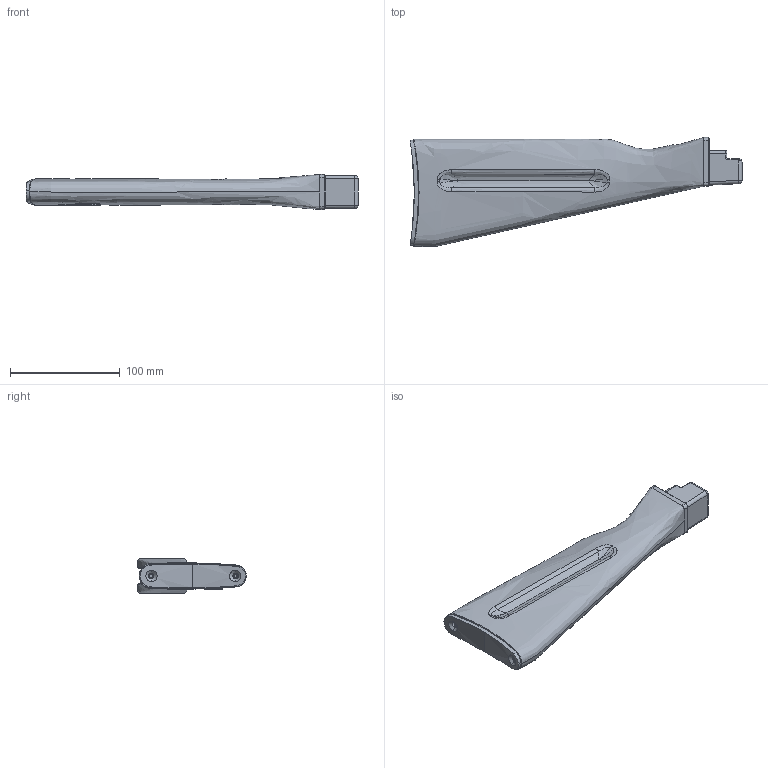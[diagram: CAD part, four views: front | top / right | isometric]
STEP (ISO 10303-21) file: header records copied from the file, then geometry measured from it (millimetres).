
FILE_DESCRIPTION (( 'STEP AP214' ), '1' );
FILE_NAME ('AK_Stock.STEP', '2013-10-08T06:17:21', ( 'elpi' ), ( '' ), 'SwSTEP 2.0', 'SolidWorks 2013', '' );
FILE_SCHEMA (( 'AUTOMOTIVE_DESIGN' ));
Length unit declared in the file: millimetre
Products named in the file (1): AK_Stock
Bounding box: 303 x 99.5 x 32 mm (x, y, z)
Volume: 405047.4 mm3; surface area: 53722.4 mm2
Topology: 1 solids, 1 shells, 163 faces, 379 edges, 228 vertices
Faces by surface type: bspline 53, cylinder 53, plane 36, torus 13, cone 6, sphere 2
Entity records: 12363 total; most frequent: CARTESIAN_POINT 8993, ORIENTED_EDGE 754, DIRECTION 603, EDGE_CURVE 377, AXIS2_PLACEMENT_3D 240, VERTEX_POINT 228, EDGE_LOOP 175, ADVANCED_FACE 163
